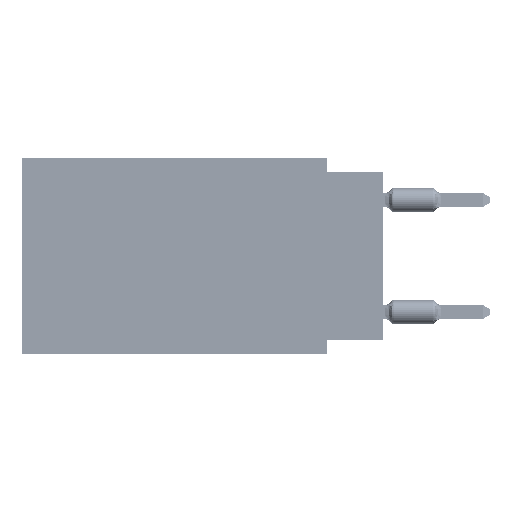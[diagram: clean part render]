
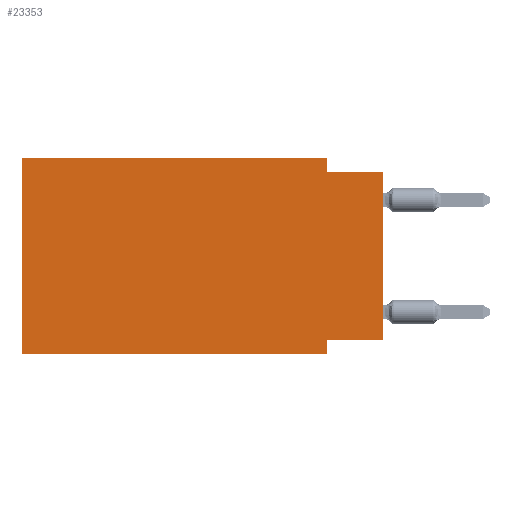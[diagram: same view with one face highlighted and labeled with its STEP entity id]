
A CAD part, left-side view. The second image highlights one B-rep face of the part: STEP entity #23353.
In plain terms, the highlighted planar face has unit normal (-1, 0, 0).
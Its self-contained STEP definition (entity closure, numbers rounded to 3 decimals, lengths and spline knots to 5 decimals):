
#76 = ORIENTED_EDGE ( 'NONE', *, *, #107038, .F. ) ;
#441 = VECTOR ( 'NONE', #114250, 39.37008 ) ;
#1832 = CARTESIAN_POINT ( 'NONE',  ( 0., 0.645, 0. ) ) ;
#1879 = CARTESIAN_POINT ( 'NONE',  ( 0., 0.1, 0. ) ) ;
#3198 = CARTESIAN_POINT ( 'NONE',  ( 0., 0.645, 0. ) ) ;
#5891 = ORIENTED_EDGE ( 'NONE', *, *, #58807, .F. ) ;
#5980 = CARTESIAN_POINT ( 'NONE',  ( 0., 0.1, -0.025 ) ) ;
#10186 = DIRECTION ( 'NONE',  ( 0., -1., 0. ) ) ;
#11279 = DIRECTION ( 'NONE',  ( 0., -1., 0. ) ) ;
#11952 = CARTESIAN_POINT ( 'NONE',  ( 0., 0.645, 0. ) ) ;
#13627 = VERTEX_POINT ( 'NONE', #3198 ) ;
#14475 = VERTEX_POINT ( 'NONE', #113002 ) ;
#18123 = DIRECTION ( 'NONE',  ( 0., 0., 1. ) ) ;
#18187 = ORIENTED_EDGE ( 'NONE', *, *, #33242, .F. ) ;
#18866 = CARTESIAN_POINT ( 'NONE',  ( 0., 0.1, -0.35 ) ) ;
#21270 = VECTOR ( 'NONE', #10186, 39.37008 ) ;
#22592 = ORIENTED_EDGE ( 'NONE', *, *, #102781, .F. ) ;
#23353 = ADVANCED_FACE ( 'NONE', ( #85153 ), #111900, .F. ) ;
#24672 = DIRECTION ( 'NONE',  ( 0., 0., 1. ) ) ;
#26929 = DIRECTION ( 'NONE',  ( 0., 1., 0. ) ) ;
#27276 = VERTEX_POINT ( 'NONE', #110922 ) ;
#30325 = CARTESIAN_POINT ( 'NONE',  ( 0., 0., -0.025 ) ) ;
#31399 = EDGE_CURVE ( 'NONE', #13627, #59679, #48471, .T. ) ;
#33242 = EDGE_CURVE ( 'NONE', #27276, #76291, #101151, .T. ) ;
#33965 = LINE ( 'NONE', #73483, #45105 ) ;
#35609 = CARTESIAN_POINT ( 'NONE',  ( 0., 0.645, 0. ) ) ;
#36838 = ORIENTED_EDGE ( 'NONE', *, *, #42997, .T. ) ;
#39530 = CARTESIAN_POINT ( 'NONE',  ( 0., 0.1, -0.35 ) ) ;
#41592 = ORIENTED_EDGE ( 'NONE', *, *, #112180, .F. ) ;
#42497 = VECTOR ( 'NONE', #94871, 39.37008 ) ;
#42997 = EDGE_CURVE ( 'NONE', #14475, #94307, #86657, .T. ) ;
#45105 = VECTOR ( 'NONE', #18123, 39.37008 ) ;
#45809 = CARTESIAN_POINT ( 'NONE',  ( 0., 0., -0.325 ) ) ;
#48471 = LINE ( 'NONE', #11952, #21270 ) ;
#50534 = VERTEX_POINT ( 'NONE', #5980 ) ;
#54326 = AXIS2_PLACEMENT_3D ( 'NONE', #1832, #56572, #63896 ) ;
#56572 = DIRECTION ( 'NONE',  ( 1., 0., 0. ) ) ;
#58807 = EDGE_CURVE ( 'NONE', #76291, #94307, #66301, .T. ) ;
#59679 = VERTEX_POINT ( 'NONE', #95607 ) ;
#63896 = DIRECTION ( 'NONE',  ( 0., 0., -1. ) ) ;
#66301 = LINE ( 'NONE', #18866, #42497 ) ;
#73483 = CARTESIAN_POINT ( 'NONE',  ( 0., 0., 0. ) ) ;
#76291 = VERTEX_POINT ( 'NONE', #115499 ) ;
#77550 = CARTESIAN_POINT ( 'NONE',  ( 0., 0.645, -0.35 ) ) ;
#80014 = ORIENTED_EDGE ( 'NONE', *, *, #31399, .F. ) ;
#82749 = CARTESIAN_POINT ( 'NONE',  ( 0., 0., -0.025 ) ) ;
#83025 = VERTEX_POINT ( 'NONE', #82749 ) ;
#85153 = FACE_OUTER_BOUND ( 'NONE', #91117, .T. ) ;
#86657 = LINE ( 'NONE', #77550, #106047 ) ;
#91117 = EDGE_LOOP ( 'NONE', ( #91163, #76, #22592, #80014, #41592, #36838, #5891, #18187 ) ) ;
#91163 = ORIENTED_EDGE ( 'NONE', *, *, #98065, .T. ) ;
#92530 = VECTOR ( 'NONE', #24672, 39.37008 ) ;
#94307 = VERTEX_POINT ( 'NONE', #39530 ) ;
#94871 = DIRECTION ( 'NONE',  ( 0., 0., -1. ) ) ;
#95607 = CARTESIAN_POINT ( 'NONE',  ( 0., 0.1, 0. ) ) ;
#96029 = LINE ( 'NONE', #30325, #441 ) ;
#96694 = DIRECTION ( 'NONE',  ( 0., 0., -1. ) ) ;
#98065 = EDGE_CURVE ( 'NONE', #27276, #83025, #33965, .T. ) ;
#101151 = LINE ( 'NONE', #45809, #103487 ) ;
#102781 = EDGE_CURVE ( 'NONE', #59679, #50534, #103420, .T. ) ;
#103420 = LINE ( 'NONE', #1879, #117469 ) ;
#103487 = VECTOR ( 'NONE', #26929, 39.37008 ) ;
#106047 = VECTOR ( 'NONE', #11279, 39.37008 ) ;
#107038 = EDGE_CURVE ( 'NONE', #50534, #83025, #96029, .T. ) ;
#110922 = CARTESIAN_POINT ( 'NONE',  ( 0., 0., -0.325 ) ) ;
#111900 = PLANE ( 'NONE',  #54326 ) ;
#112180 = EDGE_CURVE ( 'NONE', #14475, #13627, #118926, .T. ) ;
#113002 = CARTESIAN_POINT ( 'NONE',  ( 0., 0.645, -0.35 ) ) ;
#114250 = DIRECTION ( 'NONE',  ( 0., -1., 0. ) ) ;
#115499 = CARTESIAN_POINT ( 'NONE',  ( 0., 0.1, -0.325 ) ) ;
#117469 = VECTOR ( 'NONE', #96694, 39.37008 ) ;
#118926 = LINE ( 'NONE', #35609, #92530 ) ;
